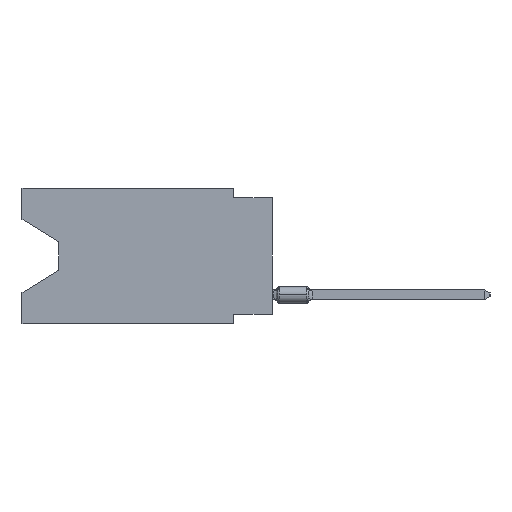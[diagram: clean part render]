
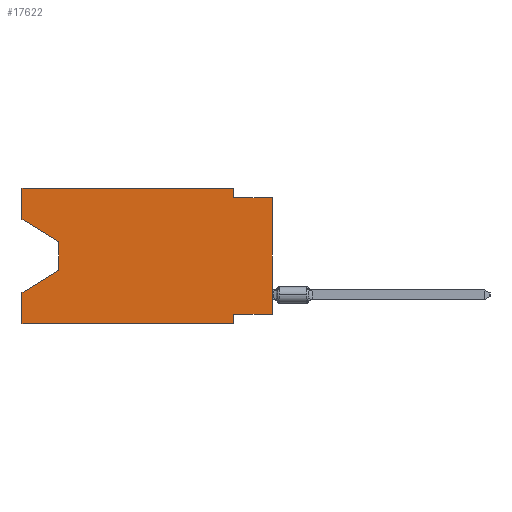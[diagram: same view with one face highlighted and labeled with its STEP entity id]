
A CAD part, left-side view. The second image highlights one B-rep face of the part: STEP entity #17622.
In plain terms, the highlighted planar face has unit normal (-1, 0, 0).
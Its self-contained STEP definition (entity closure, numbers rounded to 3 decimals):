
#149 = LINE ( 'NONE', #3869, #25361 ) ;
#469 = DIRECTION ( 'NONE',  ( 0., 0., -1. ) ) ;
#1211 = PLANE ( 'NONE',  #40316 ) ;
#1784 = DIRECTION ( 'NONE',  ( 0., -1., 0. ) ) ;
#2117 = CARTESIAN_POINT ( 'NONE',  ( 0., 13.97, -5.385 ) ) ;
#2230 = CARTESIAN_POINT ( 'NONE',  ( 0., 16.383, -2.038 ) ) ;
#2395 = CARTESIAN_POINT ( 'NONE',  ( 0., 16.383, 0. ) ) ;
#2791 = CARTESIAN_POINT ( 'NONE',  ( 0., 16.383, 0. ) ) ;
#3869 = CARTESIAN_POINT ( 'NONE',  ( 0., 2.54, 0. ) ) ;
#4186 = LINE ( 'NONE', #26033, #40886 ) ;
#5416 = LINE ( 'NONE', #19593, #28747 ) ;
#5492 = DIRECTION ( 'NONE',  ( 0., -0.855, -0.519 ) ) ;
#6317 = VECTOR ( 'NONE', #26746, 1000. ) ;
#6644 = EDGE_CURVE ( 'NONE', #24774, #23619, #12488, .T. ) ;
#6965 = ORIENTED_EDGE ( 'NONE', *, *, #12735, .F. ) ;
#7162 = CARTESIAN_POINT ( 'NONE',  ( 0., 13.97, -3.505 ) ) ;
#7907 = VERTEX_POINT ( 'NONE', #15699 ) ;
#9198 = VERTEX_POINT ( 'NONE', #11739 ) ;
#9629 = VERTEX_POINT ( 'NONE', #26780 ) ;
#11565 = EDGE_CURVE ( 'NONE', #32991, #19380, #37116, .T. ) ;
#11739 = CARTESIAN_POINT ( 'NONE',  ( 0., 0., -8.255 ) ) ;
#11918 = FACE_OUTER_BOUND ( 'NONE', #23003, .T. ) ;
#12488 = LINE ( 'NONE', #26670, #16408 ) ;
#12735 = EDGE_CURVE ( 'NONE', #27950, #32991, #149, .T. ) ;
#12915 = ORIENTED_EDGE ( 'NONE', *, *, #13966, .T. ) ;
#12936 = CARTESIAN_POINT ( 'NONE',  ( 0., 16.383, -2.038 ) ) ;
#12988 = ORIENTED_EDGE ( 'NONE', *, *, #34773, .F. ) ;
#13783 = VECTOR ( 'NONE', #45086, 1000. ) ;
#13966 = EDGE_CURVE ( 'NONE', #15689, #29993, #15958, .T. ) ;
#14697 = VECTOR ( 'NONE', #21659, 1000. ) ;
#15081 = VECTOR ( 'NONE', #5492, 1000. ) ;
#15689 = VERTEX_POINT ( 'NONE', #2230 ) ;
#15699 = CARTESIAN_POINT ( 'NONE',  ( 0., 2.54, -8.255 ) ) ;
#15958 = LINE ( 'NONE', #12936, #15081 ) ;
#16408 = VECTOR ( 'NONE', #32707, 1000. ) ;
#16586 = DIRECTION ( 'NONE',  ( 0., 1., 0. ) ) ;
#17488 = ORIENTED_EDGE ( 'NONE', *, *, #11565, .F. ) ;
#17622 = ADVANCED_FACE ( 'NONE', ( #11918 ), #1211, .F. ) ;
#19021 = CARTESIAN_POINT ( 'NONE',  ( 0., 2.54, -8.89 ) ) ;
#19380 = VERTEX_POINT ( 'NONE', #39062 ) ;
#19593 = CARTESIAN_POINT ( 'NONE',  ( 0., 0., -8.255 ) ) ;
#20585 = EDGE_CURVE ( 'NONE', #29993, #34797, #42266, .T. ) ;
#21641 = EDGE_CURVE ( 'NONE', #9198, #7907, #5416, .T. ) ;
#21659 = DIRECTION ( 'NONE',  ( 0., -1., 0. ) ) ;
#22132 = CARTESIAN_POINT ( 'NONE',  ( 0., 16.383, 0. ) ) ;
#22456 = ORIENTED_EDGE ( 'NONE', *, *, #42826, .T. ) ;
#22601 = VERTEX_POINT ( 'NONE', #35663 ) ;
#23003 = EDGE_LOOP ( 'NONE', ( #12915, #27303, #39554, #12988, #37704, #32725, #36704, #22456, #17488, #6965, #34780, #31143 ) ) ;
#23619 = VERTEX_POINT ( 'NONE', #19021 ) ;
#23760 = DIRECTION ( 'NONE',  ( 0., 0., 1. ) ) ;
#24774 = VERTEX_POINT ( 'NONE', #25853 ) ;
#25361 = VECTOR ( 'NONE', #28717, 1000. ) ;
#25853 = CARTESIAN_POINT ( 'NONE',  ( 0., 16.383, -8.89 ) ) ;
#25948 = VECTOR ( 'NONE', #45535, 1000. ) ;
#26033 = CARTESIAN_POINT ( 'NONE',  ( 0., 2.54, -8.89 ) ) ;
#26609 = EDGE_CURVE ( 'NONE', #34797, #22601, #33946, .T. ) ;
#26670 = CARTESIAN_POINT ( 'NONE',  ( 0., 16.383, -8.89 ) ) ;
#26746 = DIRECTION ( 'NONE',  ( 0., 0.855, -0.519 ) ) ;
#26780 = CARTESIAN_POINT ( 'NONE',  ( 0., 16.383, 0. ) ) ;
#27303 = ORIENTED_EDGE ( 'NONE', *, *, #20585, .T. ) ;
#27884 = CARTESIAN_POINT ( 'NONE',  ( 0., 0., 0. ) ) ;
#27950 = VERTEX_POINT ( 'NONE', #43506 ) ;
#28717 = DIRECTION ( 'NONE',  ( 0., 0., -1. ) ) ;
#28747 = VECTOR ( 'NONE', #16586, 1000. ) ;
#29851 = CARTESIAN_POINT ( 'NONE',  ( 0., 2.54, -0.635 ) ) ;
#29993 = VERTEX_POINT ( 'NONE', #45193 ) ;
#30409 = VECTOR ( 'NONE', #23760, 1000. ) ;
#30810 = CARTESIAN_POINT ( 'NONE',  ( 0., 0., -0.635 ) ) ;
#31143 = ORIENTED_EDGE ( 'NONE', *, *, #37589, .F. ) ;
#31159 = LINE ( 'NONE', #27884, #34025 ) ;
#32113 = LINE ( 'NONE', #35832, #14697 ) ;
#32163 = VECTOR ( 'NONE', #1784, 1000. ) ;
#32707 = DIRECTION ( 'NONE',  ( 0., -1., 0. ) ) ;
#32725 = ORIENTED_EDGE ( 'NONE', *, *, #36337, .F. ) ;
#32991 = VERTEX_POINT ( 'NONE', #29851 ) ;
#33946 = LINE ( 'NONE', #2117, #6317 ) ;
#34025 = VECTOR ( 'NONE', #45347, 1000. ) ;
#34773 = EDGE_CURVE ( 'NONE', #24774, #22601, #35135, .T. ) ;
#34780 = ORIENTED_EDGE ( 'NONE', *, *, #41491, .F. ) ;
#34797 = VERTEX_POINT ( 'NONE', #42091 ) ;
#35135 = LINE ( 'NONE', #2395, #30409 ) ;
#35663 = CARTESIAN_POINT ( 'NONE',  ( 0., 16.383, -6.852 ) ) ;
#35832 = CARTESIAN_POINT ( 'NONE',  ( 0., 16.383, 0. ) ) ;
#36337 = EDGE_CURVE ( 'NONE', #7907, #23619, #4186, .T. ) ;
#36704 = ORIENTED_EDGE ( 'NONE', *, *, #21641, .F. ) ;
#36773 = DIRECTION ( 'NONE',  ( 0., 0., -1. ) ) ;
#37116 = LINE ( 'NONE', #30810, #32163 ) ;
#37589 = EDGE_CURVE ( 'NONE', #15689, #9629, #37909, .T. ) ;
#37704 = ORIENTED_EDGE ( 'NONE', *, *, #6644, .T. ) ;
#37909 = LINE ( 'NONE', #2791, #13783 ) ;
#39062 = CARTESIAN_POINT ( 'NONE',  ( 0., 0., -0.635 ) ) ;
#39554 = ORIENTED_EDGE ( 'NONE', *, *, #26609, .T. ) ;
#40316 = AXIS2_PLACEMENT_3D ( 'NONE', #22132, #40490, #36773 ) ;
#40490 = DIRECTION ( 'NONE',  ( 1., 0., 0. ) ) ;
#40886 = VECTOR ( 'NONE', #469, 1000. ) ;
#41491 = EDGE_CURVE ( 'NONE', #9629, #27950, #32113, .T. ) ;
#42091 = CARTESIAN_POINT ( 'NONE',  ( 0., 13.97, -5.385 ) ) ;
#42266 = LINE ( 'NONE', #7162, #25948 ) ;
#42826 = EDGE_CURVE ( 'NONE', #9198, #19380, #31159, .T. ) ;
#43506 = CARTESIAN_POINT ( 'NONE',  ( 0., 2.54, 0. ) ) ;
#45086 = DIRECTION ( 'NONE',  ( 0., 0., 1. ) ) ;
#45193 = CARTESIAN_POINT ( 'NONE',  ( 0., 13.97, -3.505 ) ) ;
#45347 = DIRECTION ( 'NONE',  ( 0., 0., 1. ) ) ;
#45535 = DIRECTION ( 'NONE',  ( 0., 0., -1. ) ) ;
